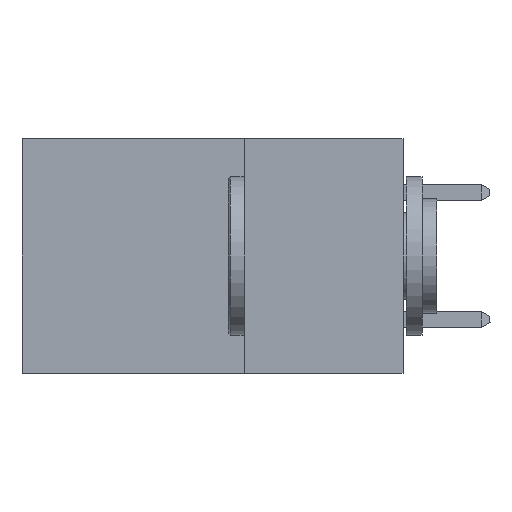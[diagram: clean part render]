
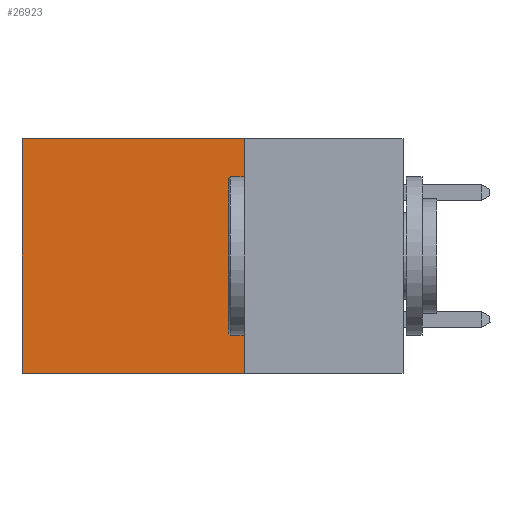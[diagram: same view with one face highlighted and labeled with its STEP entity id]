
A CAD part, left-side view. The second image highlights one B-rep face of the part: STEP entity #26923.
In plain terms, the highlighted planar face has unit normal (-1, 0, 0).
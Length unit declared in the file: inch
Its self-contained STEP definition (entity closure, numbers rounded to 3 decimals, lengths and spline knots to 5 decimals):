
#31 = ORIENTED_EDGE ( 'NONE', *, *, #8150, .T. ) ;
#54 = ORIENTED_EDGE ( 'NONE', *, *, #17908, .F. ) ;
#2091 = CARTESIAN_POINT ( 'NONE',  ( 0.2875, 0.25, 0. ) ) ;
#5252 = FACE_OUTER_BOUND ( 'NONE', #28075, .T. ) ;
#5890 = VERTEX_POINT ( 'NONE', #2091 ) ;
#6281 = ORIENTED_EDGE ( 'NONE', *, *, #19025, .T. ) ;
#7325 = CARTESIAN_POINT ( 'NONE',  ( 0.2875, 0.25, -0.37 ) ) ;
#7446 = CARTESIAN_POINT ( 'NONE',  ( 0.2875, 0.25, 0. ) ) ;
#8120 = CARTESIAN_POINT ( 'NONE',  ( 0.2875, 0.25, 0. ) ) ;
#8150 = EDGE_CURVE ( 'NONE', #5890, #28063, #28850, .T. ) ;
#8264 = VECTOR ( 'NONE', #25457, 39.37008 ) ;
#11111 = LINE ( 'NONE', #14071, #16203 ) ;
#11251 = CARTESIAN_POINT ( 'NONE',  ( 0.2875, 0.25, -0.37 ) ) ;
#11575 = VERTEX_POINT ( 'NONE', #25548 ) ;
#14071 = CARTESIAN_POINT ( 'NONE',  ( 0.2875, 0.25, 0. ) ) ;
#14376 = VECTOR ( 'NONE', #18404, 39.37008 ) ;
#15112 = EDGE_CURVE ( 'NONE', #5890, #16891, #11111, .T. ) ;
#15759 = LINE ( 'NONE', #11251, #20118 ) ;
#16156 = DIRECTION ( 'NONE',  ( 0., 1., 0. ) ) ;
#16203 = VECTOR ( 'NONE', #24118, 39.37008 ) ;
#16891 = VERTEX_POINT ( 'NONE', #7325 ) ;
#17719 = ORIENTED_EDGE ( 'NONE', *, *, #15112, .F. ) ;
#17908 = EDGE_CURVE ( 'NONE', #16891, #11575, #15759, .T. ) ;
#18023 = CARTESIAN_POINT ( 'NONE',  ( 0.2875, 0.6, 0. ) ) ;
#18404 = DIRECTION ( 'NONE',  ( 0., 1., 0. ) ) ;
#19025 = EDGE_CURVE ( 'NONE', #28063, #11575, #29401, .T. ) ;
#19315 = CARTESIAN_POINT ( 'NONE',  ( 0.2875, 0.6, 0. ) ) ;
#20118 = VECTOR ( 'NONE', #16156, 39.37008 ) ;
#22273 = DIRECTION ( 'NONE',  ( 1., 0., 0. ) ) ;
#24118 = DIRECTION ( 'NONE',  ( 0., 0., -1. ) ) ;
#24702 = PLANE ( 'NONE',  #25241 ) ;
#25241 = AXIS2_PLACEMENT_3D ( 'NONE', #7446, #22273, #29701 ) ;
#25457 = DIRECTION ( 'NONE',  ( 0., 0., -1. ) ) ;
#25548 = CARTESIAN_POINT ( 'NONE',  ( 0.2875, 0.6, -0.37 ) ) ;
#26923 = ADVANCED_FACE ( 'NONE', ( #5252 ), #24702, .F. ) ;
#28063 = VERTEX_POINT ( 'NONE', #19315 ) ;
#28075 = EDGE_LOOP ( 'NONE', ( #6281, #54, #17719, #31 ) ) ;
#28850 = LINE ( 'NONE', #8120, #14376 ) ;
#29401 = LINE ( 'NONE', #18023, #8264 ) ;
#29701 = DIRECTION ( 'NONE',  ( 0., 0., -1. ) ) ;
